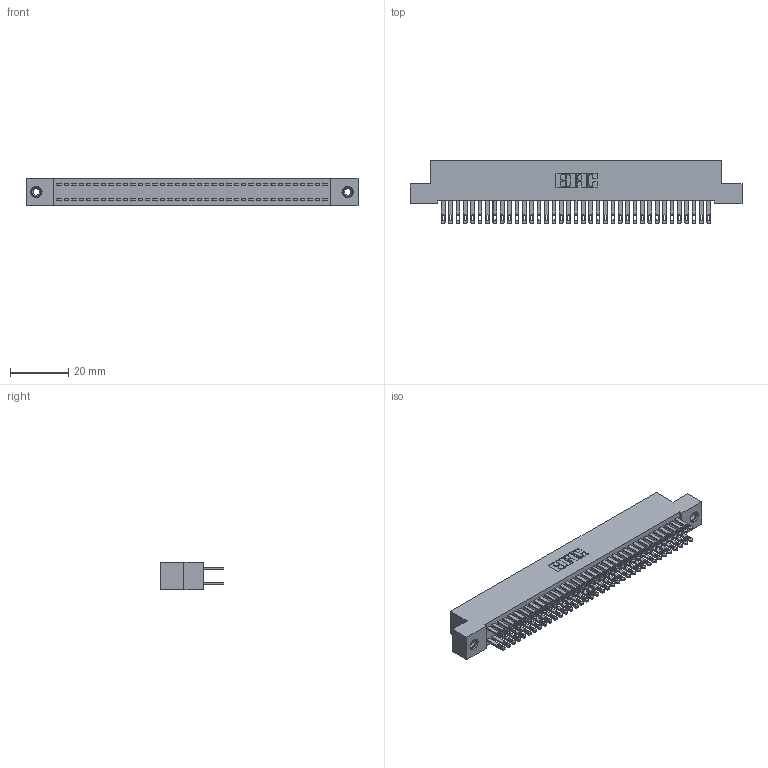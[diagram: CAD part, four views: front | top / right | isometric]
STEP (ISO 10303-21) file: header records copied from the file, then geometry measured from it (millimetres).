
FILE_DESCRIPTION (( 'STEP AP203' ), '1' );
FILE_NAME ('342-074-500-208.STEP', '2019-10-03T17:00:39', ( '' ), ( '' ), 'SwSTEP 2.0', 'SolidWorks 2016', '' );
FILE_SCHEMA (( 'CONFIG_CONTROL_DESIGN' ));
Length unit declared in the file: inch
Products named in the file (4): 342 Part_TI; 345-292-001_345-293-100; 345-250-001_345-250-003-102; 342-074-500-208
Assembly tree (77 placements, depth 2):
  342-074-500-208
    342 Part_TI
    345-292-001_345-293-100  x74
    345-250-001_345-250-003-102  x2
Bounding box: 114.3 x 21.85 x 9.4 mm (x, y, z)
Volume: 10466.6 mm3; surface area: 17632.6 mm2
Topology: 77 solids, 77 shells, 3722 faces, 11313 edges, 7534 vertices
Faces by surface type: plane 2318, cylinder 1388, cone 12, torus 4
Entity records: 25434 total; most frequent: CARTESIAN_POINT 4201, ORIENTED_EDGE 4130, DIRECTION 3631, EDGE_CURVE 2065, VECTOR 1913, LINE 1913, VERTEX_POINT 1372, AXIS2_PLACEMENT_3D 859
